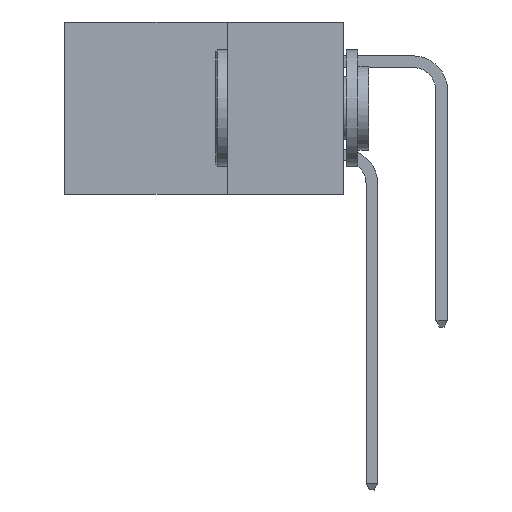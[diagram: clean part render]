
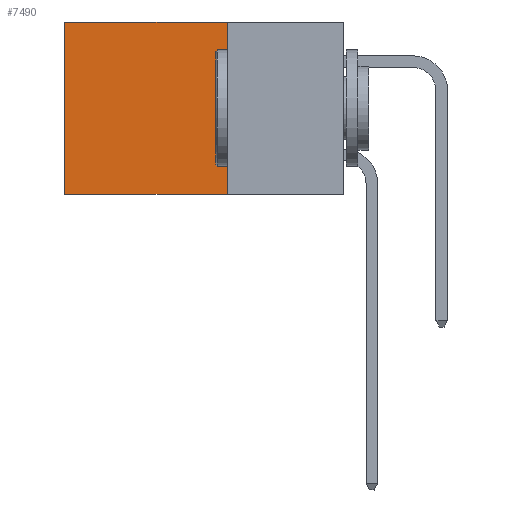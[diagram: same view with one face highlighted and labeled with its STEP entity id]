
A CAD part, left-side view. The second image highlights one B-rep face of the part: STEP entity #7490.
In plain terms, the highlighted planar face has unit normal (-1, 0, 0).
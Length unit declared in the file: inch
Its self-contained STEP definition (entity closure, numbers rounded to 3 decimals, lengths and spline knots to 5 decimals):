
#120 = VECTOR ( 'NONE', #7941, 39.37008 ) ;
#719 = EDGE_LOOP ( 'NONE', ( #1404, #1694, #6841, #1459 ) ) ;
#892 = CARTESIAN_POINT ( 'NONE',  ( 0.2615, 0.25, 0. ) ) ;
#1404 = ORIENTED_EDGE ( 'NONE', *, *, #6606, .T. ) ;
#1413 = FACE_OUTER_BOUND ( 'NONE', #719, .T. ) ;
#1459 = ORIENTED_EDGE ( 'NONE', *, *, #3329, .T. ) ;
#1475 = DIRECTION ( 'NONE',  ( 0., 0., -1. ) ) ;
#1694 = ORIENTED_EDGE ( 'NONE', *, *, #2384, .F. ) ;
#2035 = VERTEX_POINT ( 'NONE', #2290 ) ;
#2048 = CARTESIAN_POINT ( 'NONE',  ( 0.2615, 0.6, 0. ) ) ;
#2290 = CARTESIAN_POINT ( 'NONE',  ( 0.2615, 0.6, -0.37 ) ) ;
#2384 = EDGE_CURVE ( 'NONE', #10443, #2035, #3075, .T. ) ;
#2714 = VECTOR ( 'NONE', #10284, 39.37008 ) ;
#3073 = CARTESIAN_POINT ( 'NONE',  ( 0.2615, 0.6, -0.37 ) ) ;
#3075 = LINE ( 'NONE', #10177, #2714 ) ;
#3101 = VERTEX_POINT ( 'NONE', #9918 ) ;
#3277 = DIRECTION ( 'NONE',  ( 0., 0., -1. ) ) ;
#3329 = EDGE_CURVE ( 'NONE', #3101, #5465, #6247, .T. ) ;
#4966 = CARTESIAN_POINT ( 'NONE',  ( 0.2615, 0.25, -0.37 ) ) ;
#5195 = LINE ( 'NONE', #4966, #11423 ) ;
#5465 = VERTEX_POINT ( 'NONE', #2048 ) ;
#5821 = PLANE ( 'NONE',  #11245 ) ;
#5889 = DIRECTION ( 'NONE',  ( 1., 0., 0. ) ) ;
#6247 = LINE ( 'NONE', #892, #120 ) ;
#6606 = EDGE_CURVE ( 'NONE', #5465, #2035, #11025, .T. ) ;
#6617 = DIRECTION ( 'NONE',  ( 0., 0., -1. ) ) ;
#6841 = ORIENTED_EDGE ( 'NONE', *, *, #7514, .F. ) ;
#7490 = ADVANCED_FACE ( 'NONE', ( #1413 ), #5821, .F. ) ;
#7514 = EDGE_CURVE ( 'NONE', #3101, #10443, #5195, .T. ) ;
#7941 = DIRECTION ( 'NONE',  ( 0., 1., 0. ) ) ;
#8189 = CARTESIAN_POINT ( 'NONE',  ( 0.2615, 0.25, -0.37 ) ) ;
#9918 = CARTESIAN_POINT ( 'NONE',  ( 0.2615, 0.25, 0. ) ) ;
#9932 = VECTOR ( 'NONE', #6617, 39.37008 ) ;
#10177 = CARTESIAN_POINT ( 'NONE',  ( 0.2615, 0.25, -0.37 ) ) ;
#10284 = DIRECTION ( 'NONE',  ( 0., 1., 0. ) ) ;
#10443 = VERTEX_POINT ( 'NONE', #8189 ) ;
#11025 = LINE ( 'NONE', #3073, #9932 ) ;
#11175 = CARTESIAN_POINT ( 'NONE',  ( 0.2615, 0.25, -0.37 ) ) ;
#11245 = AXIS2_PLACEMENT_3D ( 'NONE', #11175, #5889, #1475 ) ;
#11423 = VECTOR ( 'NONE', #3277, 39.37008 ) ;
